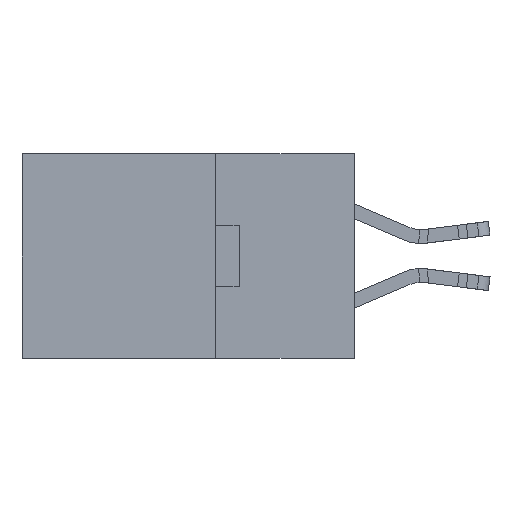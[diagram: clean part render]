
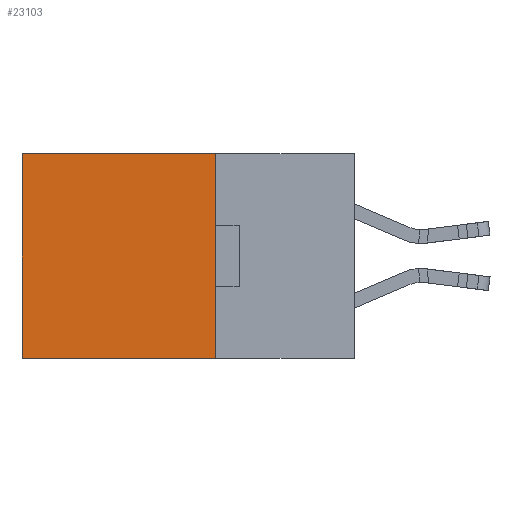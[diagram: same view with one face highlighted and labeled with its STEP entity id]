
A CAD part, left-side view. The second image highlights one B-rep face of the part: STEP entity #23103.
In plain terms, the highlighted planar face has unit normal (-1, 0, 0).
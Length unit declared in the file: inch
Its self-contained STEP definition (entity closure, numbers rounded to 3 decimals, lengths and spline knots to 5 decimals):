
#5 = CARTESIAN_POINT ( 'NONE',  ( 0.2615, 0.25, -0.37 ) ) ;
#487 = CARTESIAN_POINT ( 'NONE',  ( 0.2615, 0.6, 0. ) ) ;
#809 = DIRECTION ( 'NONE',  ( 0., 0., -1. ) ) ;
#2033 = VECTOR ( 'NONE', #13566, 39.37008 ) ;
#2237 = VERTEX_POINT ( 'NONE', #5 ) ;
#2960 = LINE ( 'NONE', #24734, #20293 ) ;
#3079 = CARTESIAN_POINT ( 'NONE',  ( 0.2615, 0.25, 0. ) ) ;
#4543 = DIRECTION ( 'NONE',  ( 0., 1., 0. ) ) ;
#5209 = EDGE_CURVE ( 'NONE', #9879, #10964, #23607, .T. ) ;
#5924 = ORIENTED_EDGE ( 'NONE', *, *, #11569, .F. ) ;
#6592 = VECTOR ( 'NONE', #9197, 39.37008 ) ;
#7819 = ORIENTED_EDGE ( 'NONE', *, *, #11513, .T. ) ;
#8906 = EDGE_CURVE ( 'NONE', #2237, #12219, #2960, .T. ) ;
#8948 = AXIS2_PLACEMENT_3D ( 'NONE', #27733, #14320, #809 ) ;
#9197 = DIRECTION ( 'NONE',  ( 0., 0., -1. ) ) ;
#9344 = ORIENTED_EDGE ( 'NONE', *, *, #5209, .T. ) ;
#9879 = VERTEX_POINT ( 'NONE', #21379 ) ;
#10964 = VERTEX_POINT ( 'NONE', #487 ) ;
#11513 = EDGE_CURVE ( 'NONE', #10964, #12219, #12595, .T. ) ;
#11569 = EDGE_CURVE ( 'NONE', #9879, #2237, #23157, .T. ) ;
#12219 = VERTEX_POINT ( 'NONE', #24739 ) ;
#12337 = VECTOR ( 'NONE', #21151, 39.37008 ) ;
#12595 = LINE ( 'NONE', #26994, #2033 ) ;
#13566 = DIRECTION ( 'NONE',  ( 0., 0., -1. ) ) ;
#14320 = DIRECTION ( 'NONE',  ( 1., 0., 0. ) ) ;
#18819 = PLANE ( 'NONE',  #8948 ) ;
#19133 = EDGE_LOOP ( 'NONE', ( #7819, #28130, #5924, #9344 ) ) ;
#20293 = VECTOR ( 'NONE', #4543, 39.37008 ) ;
#21151 = DIRECTION ( 'NONE',  ( 0., 1., 0. ) ) ;
#21379 = CARTESIAN_POINT ( 'NONE',  ( 0.2615, 0.25, 0. ) ) ;
#23103 = ADVANCED_FACE ( 'NONE', ( #28173 ), #18819, .F. ) ;
#23157 = LINE ( 'NONE', #24961, #6592 ) ;
#23607 = LINE ( 'NONE', #3079, #12337 ) ;
#24734 = CARTESIAN_POINT ( 'NONE',  ( 0.2615, 0.25, -0.37 ) ) ;
#24739 = CARTESIAN_POINT ( 'NONE',  ( 0.2615, 0.6, -0.37 ) ) ;
#24961 = CARTESIAN_POINT ( 'NONE',  ( 0.2615, 0.25, -0.37 ) ) ;
#26994 = CARTESIAN_POINT ( 'NONE',  ( 0.2615, 0.6, -0.37 ) ) ;
#27733 = CARTESIAN_POINT ( 'NONE',  ( 0.2615, 0.25, -0.37 ) ) ;
#28130 = ORIENTED_EDGE ( 'NONE', *, *, #8906, .F. ) ;
#28173 = FACE_OUTER_BOUND ( 'NONE', #19133, .T. ) ;
